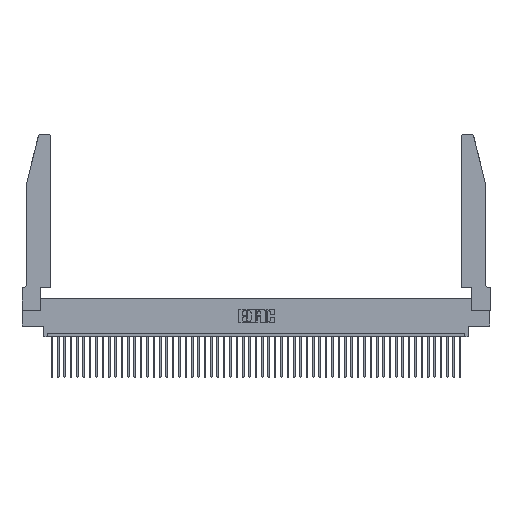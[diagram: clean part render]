
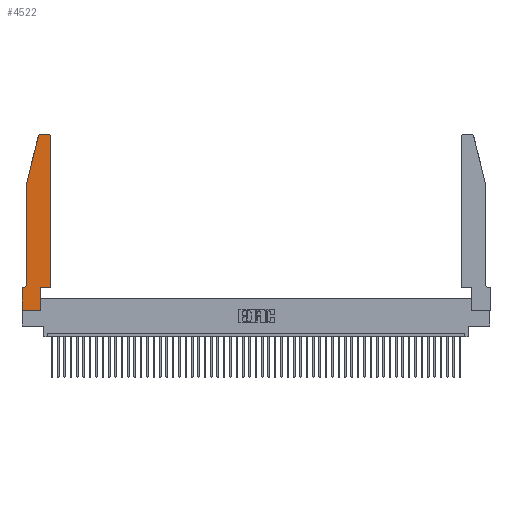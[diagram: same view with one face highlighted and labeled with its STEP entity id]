
A CAD part, top view. The second image highlights one B-rep face of the part: STEP entity #4522.
In plain terms, the highlighted planar face has unit normal (0, 0, 1).
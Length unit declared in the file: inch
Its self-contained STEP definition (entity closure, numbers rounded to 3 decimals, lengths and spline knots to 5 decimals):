
#619 = AXIS2_PLACEMENT_3D ( 'NONE', #29394, #41188, #9524 ) ;
#1165 = VERTEX_POINT ( 'NONE', #23733 ) ;
#2304 = DIRECTION ( 'NONE',  ( 1., 0., 0. ) ) ;
#2840 = CARTESIAN_POINT ( 'NONE',  ( 0.2865, 0.35, 0.37 ) ) ;
#3013 = CARTESIAN_POINT ( 'NONE',  ( 0.4505, 0.35, 0.37 ) ) ;
#3705 = VECTOR ( 'NONE', #4321, 39.37008 ) ;
#4321 = DIRECTION ( 'NONE',  ( -1., 0., 0. ) ) ;
#4522 = ADVANCED_FACE ( 'NONE', ( #35759 ), #25149, .T. ) ;
#4583 = CARTESIAN_POINT ( 'NONE',  ( 0.4505, 0.35, 0.37 ) ) ;
#5699 = CARTESIAN_POINT ( 'NONE',  ( 0.0755, 0.42, 0.37 ) ) ;
#5742 = CARTESIAN_POINT ( 'NONE',  ( 0.4505, 2.72, 0.37 ) ) ;
#6321 = LINE ( 'NONE', #11867, #22242 ) ;
#6330 = CARTESIAN_POINT ( 'NONE',  ( 0.4205, 2.72, 0.37 ) ) ;
#6506 = VERTEX_POINT ( 'NONE', #5699 ) ;
#7143 = CARTESIAN_POINT ( 'NONE',  ( 0.0055, 0.42, 0.37 ) ) ;
#7618 = DIRECTION ( 'NONE',  ( -1., 0., 0. ) ) ;
#7766 = DIRECTION ( 'NONE',  ( 0., -1., 0. ) ) ;
#7772 = EDGE_CURVE ( 'NONE', #8536, #6506, #6321, .T. ) ;
#7969 = DIRECTION ( 'NONE',  ( -1., 0., 0. ) ) ;
#8347 = ORIENTED_EDGE ( 'NONE', *, *, #38986, .T. ) ;
#8536 = VERTEX_POINT ( 'NONE', #25483 ) ;
#9524 = DIRECTION ( 'NONE',  ( 1., 0., 0. ) ) ;
#10297 = CARTESIAN_POINT ( 'NONE',  ( 0.284, 2.75, 0.37 ) ) ;
#10860 = ORIENTED_EDGE ( 'NONE', *, *, #18692, .T. ) ;
#10935 = EDGE_CURVE ( 'NONE', #1165, #24368, #23816, .T. ) ;
#11615 = LINE ( 'NONE', #2840, #15304 ) ;
#11867 = CARTESIAN_POINT ( 'NONE',  ( 0.0755, 2., 0.37 ) ) ;
#12019 = CARTESIAN_POINT ( 'NONE',  ( 0.2865, 0.35, 0.37 ) ) ;
#12940 = EDGE_CURVE ( 'NONE', #35860, #50698, #11615, .T. ) ;
#12995 = EDGE_CURVE ( 'NONE', #49912, #50367, #16533, .T. ) ;
#13358 = VECTOR ( 'NONE', #33687, 39.37008 ) ;
#13642 = CIRCLE ( 'NONE', #619, 0.03 ) ;
#13983 = DIRECTION ( 'NONE',  ( 0., 1., 0. ) ) ;
#14293 = ORIENTED_EDGE ( 'NONE', *, *, #29567, .T. ) ;
#14374 = DIRECTION ( 'NONE',  ( 0., 0., 1. ) ) ;
#15304 = VECTOR ( 'NONE', #26528, 39.37008 ) ;
#15311 = EDGE_CURVE ( 'NONE', #50698, #49912, #37093, .T. ) ;
#15429 = VERTEX_POINT ( 'NONE', #10297 ) ;
#15481 = CARTESIAN_POINT ( 'NONE',  ( 0.0755, 0.35, 0.37 ) ) ;
#16533 = LINE ( 'NONE', #3013, #17112 ) ;
#16545 = EDGE_CURVE ( 'NONE', #15429, #42155, #13642, .T. ) ;
#17112 = VECTOR ( 'NONE', #13983, 39.37008 ) ;
#18692 = EDGE_CURVE ( 'NONE', #28290, #15429, #44743, .T. ) ;
#20323 = ORIENTED_EDGE ( 'NONE', *, *, #37960, .T. ) ;
#21294 = VECTOR ( 'NONE', #42350, 39.37008 ) ;
#21531 = CARTESIAN_POINT ( 'NONE',  ( 0., 0., 0.37 ) ) ;
#22078 = CARTESIAN_POINT ( 'NONE',  ( 0.25487, 2.72718, 0.37 ) ) ;
#22242 = VECTOR ( 'NONE', #7766, 39.37008 ) ;
#22568 = VERTEX_POINT ( 'NONE', #34289 ) ;
#23733 = CARTESIAN_POINT ( 'NONE',  ( 0., 0.35, 0.37 ) ) ;
#23816 = LINE ( 'NONE', #41364, #13358 ) ;
#24368 = VERTEX_POINT ( 'NONE', #21531 ) ;
#24454 = ORIENTED_EDGE ( 'NONE', *, *, #12940, .T. ) ;
#24516 = CARTESIAN_POINT ( 'NONE',  ( 0.4205, 2.75, 0.37 ) ) ;
#24655 = ORIENTED_EDGE ( 'NONE', *, *, #15311, .T. ) ;
#25149 = PLANE ( 'NONE',  #33125 ) ;
#25483 = CARTESIAN_POINT ( 'NONE',  ( 0.0755, 2., 0.37 ) ) ;
#26024 = DIRECTION ( 'NONE',  ( 0., 0., 1. ) ) ;
#26473 = CARTESIAN_POINT ( 'NONE',  ( 0., 0., 0.37 ) ) ;
#26528 = DIRECTION ( 'NONE',  ( 0., 1., 0. ) ) ;
#26575 = ORIENTED_EDGE ( 'NONE', *, *, #7772, .T. ) ;
#27969 = CARTESIAN_POINT ( 'NONE',  ( 0.2605, 2.75, 0.37 ) ) ;
#28110 = ORIENTED_EDGE ( 'NONE', *, *, #49781, .T. ) ;
#28290 = VERTEX_POINT ( 'NONE', #24516 ) ;
#29394 = CARTESIAN_POINT ( 'NONE',  ( 0.284, 2.72, 0.37 ) ) ;
#29567 = EDGE_CURVE ( 'NONE', #6506, #22568, #36656, .T. ) ;
#29794 = AXIS2_PLACEMENT_3D ( 'NONE', #7143, #30948, #7969 ) ;
#30138 = EDGE_LOOP ( 'NONE', ( #10860, #39570, #8347, #26575, #14293, #50438, #48211, #28110, #24454, #24655, #30965, #20323 ) ) ;
#30948 = DIRECTION ( 'NONE',  ( 0., 0., -1. ) ) ;
#30965 = ORIENTED_EDGE ( 'NONE', *, *, #12995, .T. ) ;
#32064 = VECTOR ( 'NONE', #7618, 39.37008 ) ;
#32348 = CIRCLE ( 'NONE', #50676, 0.03 ) ;
#33125 = AXIS2_PLACEMENT_3D ( 'NONE', #33220, #26024, #42247 ) ;
#33220 = CARTESIAN_POINT ( 'NONE',  ( 0., 0.35, 0.37 ) ) ;
#33687 = DIRECTION ( 'NONE',  ( 0., -1., 0. ) ) ;
#34087 = LINE ( 'NONE', #36167, #48125 ) ;
#34236 = LINE ( 'NONE', #26473, #21294 ) ;
#34289 = CARTESIAN_POINT ( 'NONE',  ( 0.0055, 0.35, 0.37 ) ) ;
#35759 = FACE_OUTER_BOUND ( 'NONE', #30138, .T. ) ;
#35839 = DIRECTION ( 'NONE',  ( -0.239, -0.971, 0. ) ) ;
#35860 = VERTEX_POINT ( 'NONE', #48621 ) ;
#36167 = CARTESIAN_POINT ( 'NONE',  ( 0.0755, 2., 0.37 ) ) ;
#36656 = CIRCLE ( 'NONE', #29794, 0.07 ) ;
#36762 = EDGE_CURVE ( 'NONE', #22568, #1165, #39406, .T. ) ;
#37093 = LINE ( 'NONE', #4583, #40760 ) ;
#37960 = EDGE_CURVE ( 'NONE', #50367, #28290, #32348, .T. ) ;
#38986 = EDGE_CURVE ( 'NONE', #42155, #8536, #34087, .T. ) ;
#39406 = LINE ( 'NONE', #15481, #32064 ) ;
#39570 = ORIENTED_EDGE ( 'NONE', *, *, #16545, .T. ) ;
#40760 = VECTOR ( 'NONE', #2304, 39.37008 ) ;
#41188 = DIRECTION ( 'NONE',  ( 0., 0., 1. ) ) ;
#41364 = CARTESIAN_POINT ( 'NONE',  ( 0., 0., 0.37 ) ) ;
#42155 = VERTEX_POINT ( 'NONE', #22078 ) ;
#42247 = DIRECTION ( 'NONE',  ( 1., 0., 0. ) ) ;
#42350 = DIRECTION ( 'NONE',  ( 1., 0., 0. ) ) ;
#44743 = LINE ( 'NONE', #27969, #3705 ) ;
#45534 = DIRECTION ( 'NONE',  ( 1., 0., 0. ) ) ;
#48125 = VECTOR ( 'NONE', #35839, 39.37008 ) ;
#48211 = ORIENTED_EDGE ( 'NONE', *, *, #10935, .T. ) ;
#48621 = CARTESIAN_POINT ( 'NONE',  ( 0.2865, 0., 0.37 ) ) ;
#49781 = EDGE_CURVE ( 'NONE', #24368, #35860, #34236, .T. ) ;
#49912 = VERTEX_POINT ( 'NONE', #50697 ) ;
#50367 = VERTEX_POINT ( 'NONE', #5742 ) ;
#50438 = ORIENTED_EDGE ( 'NONE', *, *, #36762, .T. ) ;
#50676 = AXIS2_PLACEMENT_3D ( 'NONE', #6330, #14374, #45534 ) ;
#50697 = CARTESIAN_POINT ( 'NONE',  ( 0.4505, 0.35, 0.37 ) ) ;
#50698 = VERTEX_POINT ( 'NONE', #12019 ) ;
